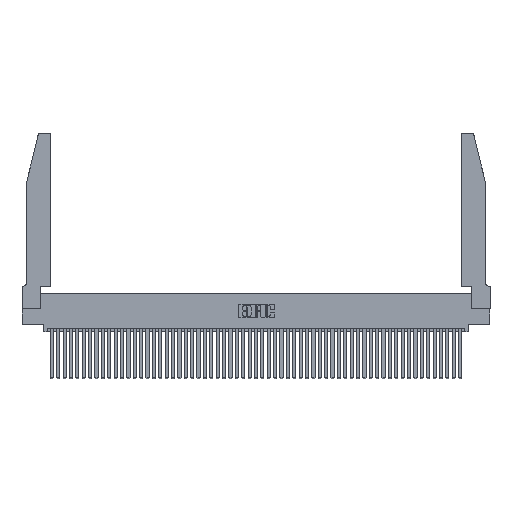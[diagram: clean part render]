
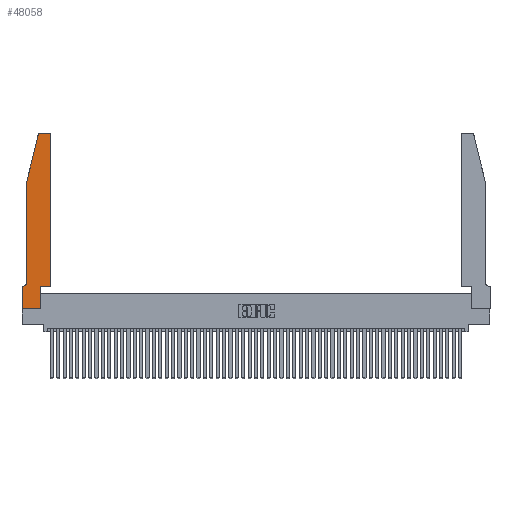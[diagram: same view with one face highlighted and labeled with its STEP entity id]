
A CAD part, top view. The second image highlights one B-rep face of the part: STEP entity #48058.
In plain terms, the highlighted planar face has unit normal (0, 0, 1).
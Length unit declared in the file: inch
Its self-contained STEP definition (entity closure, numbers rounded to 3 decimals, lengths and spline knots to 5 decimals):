
#108 = EDGE_CURVE ( 'NONE', #32407, #50588, #40248, .T. ) ;
#417 = DIRECTION ( 'NONE',  ( -1., 0., 0. ) ) ;
#1207 = EDGE_CURVE ( 'NONE', #45437, #23000, #37636, .T. ) ;
#2718 = DIRECTION ( 'NONE',  ( 1., 0., 0. ) ) ;
#3512 = CARTESIAN_POINT ( 'NONE',  ( 0.0755, 2., 0.37 ) ) ;
#3935 = VERTEX_POINT ( 'NONE', #17784 ) ;
#4068 = VECTOR ( 'NONE', #6669, 39.37008 ) ;
#4568 = DIRECTION ( 'NONE',  ( 0., 1., 0. ) ) ;
#4619 = ORIENTED_EDGE ( 'NONE', *, *, #37289, .T. ) ;
#4667 = VECTOR ( 'NONE', #39331, 39.37008 ) ;
#5758 = DIRECTION ( 'NONE',  ( 0., 0., 1. ) ) ;
#6669 = DIRECTION ( 'NONE',  ( -1., 0., 0. ) ) ;
#7235 = CARTESIAN_POINT ( 'NONE',  ( 0.0755, 0.35, 0.37 ) ) ;
#7594 = DIRECTION ( 'NONE',  ( -0.239, -0.971, 0. ) ) ;
#8000 = ORIENTED_EDGE ( 'NONE', *, *, #46721, .T. ) ;
#8265 = LINE ( 'NONE', #27307, #45809 ) ;
#9002 = LINE ( 'NONE', #36917, #34467 ) ;
#9204 = AXIS2_PLACEMENT_3D ( 'NONE', #42686, #26706, #26871 ) ;
#9353 = VECTOR ( 'NONE', #34110, 39.37008 ) ;
#9788 = LINE ( 'NONE', #3512, #52331 ) ;
#9932 = ORIENTED_EDGE ( 'NONE', *, *, #1207, .T. ) ;
#10025 = CARTESIAN_POINT ( 'NONE',  ( 0., 0., 0.37 ) ) ;
#11655 = CARTESIAN_POINT ( 'NONE',  ( 0.284, 2.75, 0.37 ) ) ;
#12198 = CARTESIAN_POINT ( 'NONE',  ( 0.0055, 0.42, 0.37 ) ) ;
#12377 = VERTEX_POINT ( 'NONE', #26930 ) ;
#12613 = EDGE_CURVE ( 'NONE', #50588, #3935, #20645, .T. ) ;
#12915 = CARTESIAN_POINT ( 'NONE',  ( 0.25487, 2.72718, 0.37 ) ) ;
#13933 = CARTESIAN_POINT ( 'NONE',  ( 0.2865, 0.35, 0.37 ) ) ;
#15765 = AXIS2_PLACEMENT_3D ( 'NONE', #12198, #24817, #417 ) ;
#15839 = ORIENTED_EDGE ( 'NONE', *, *, #20529, .T. ) ;
#17040 = EDGE_CURVE ( 'NONE', #39948, #32407, #26724, .T. ) ;
#17784 = CARTESIAN_POINT ( 'NONE',  ( 0.2865, 0., 0.37 ) ) ;
#18022 = AXIS2_PLACEMENT_3D ( 'NONE', #27081, #30800, #2718 ) ;
#18145 = CARTESIAN_POINT ( 'NONE',  ( 0.4205, 2.75, 0.37 ) ) ;
#19070 = PLANE ( 'NONE',  #18022 ) ;
#19079 = CARTESIAN_POINT ( 'NONE',  ( 0.2605, 2.75, 0.37 ) ) ;
#19269 = CARTESIAN_POINT ( 'NONE',  ( 0., 0., 0.37 ) ) ;
#20529 = EDGE_CURVE ( 'NONE', #36280, #29135, #9788, .T. ) ;
#20645 = LINE ( 'NONE', #19269, #34631 ) ;
#21589 = DIRECTION ( 'NONE',  ( 0., 1., 0. ) ) ;
#21901 = ORIENTED_EDGE ( 'NONE', *, *, #52190, .T. ) ;
#23000 = VERTEX_POINT ( 'NONE', #18145 ) ;
#23869 = CARTESIAN_POINT ( 'NONE',  ( 0.0755, 0.42, 0.37 ) ) ;
#24288 = CARTESIAN_POINT ( 'NONE',  ( 0.4505, 0.35, 0.37 ) ) ;
#24817 = DIRECTION ( 'NONE',  ( 0., 0., -1. ) ) ;
#26064 = VECTOR ( 'NONE', #51990, 39.37008 ) ;
#26697 = CARTESIAN_POINT ( 'NONE',  ( 0.284, 2.72, 0.37 ) ) ;
#26706 = DIRECTION ( 'NONE',  ( 0., 0., 1. ) ) ;
#26724 = LINE ( 'NONE', #7235, #26064 ) ;
#26871 = DIRECTION ( 'NONE',  ( 1., 0., 0. ) ) ;
#26930 = CARTESIAN_POINT ( 'NONE',  ( 0.2865, 0.35, 0.37 ) ) ;
#27081 = CARTESIAN_POINT ( 'NONE',  ( 0., 0.35, 0.37 ) ) ;
#27307 = CARTESIAN_POINT ( 'NONE',  ( 0.4505, 0.35, 0.37 ) ) ;
#27443 = DIRECTION ( 'NONE',  ( 1., 0., 0. ) ) ;
#28082 = ORIENTED_EDGE ( 'NONE', *, *, #108, .T. ) ;
#29135 = VERTEX_POINT ( 'NONE', #40677 ) ;
#29564 = CIRCLE ( 'NONE', #15765, 0.07 ) ;
#29857 = EDGE_CURVE ( 'NONE', #3935, #12377, #48520, .T. ) ;
#30345 = LINE ( 'NONE', #50435, #9353 ) ;
#30800 = DIRECTION ( 'NONE',  ( 0., 0., 1. ) ) ;
#31534 = DIRECTION ( 'NONE',  ( 1., 0., 0. ) ) ;
#32015 = CARTESIAN_POINT ( 'NONE',  ( 0.0055, 0.35, 0.37 ) ) ;
#32407 = VERTEX_POINT ( 'NONE', #50140 ) ;
#33489 = EDGE_CURVE ( 'NONE', #52221, #45437, #9002, .T. ) ;
#33830 = ORIENTED_EDGE ( 'NONE', *, *, #17040, .T. ) ;
#34055 = VERTEX_POINT ( 'NONE', #11655 ) ;
#34110 = DIRECTION ( 'NONE',  ( 0., -1., 0. ) ) ;
#34467 = VECTOR ( 'NONE', #4568, 39.37008 ) ;
#34631 = VECTOR ( 'NONE', #27443, 39.37008 ) ;
#35335 = CARTESIAN_POINT ( 'NONE',  ( 0.4505, 2.72, 0.37 ) ) ;
#36280 = VERTEX_POINT ( 'NONE', #12915 ) ;
#36613 = ORIENTED_EDGE ( 'NONE', *, *, #12613, .T. ) ;
#36917 = CARTESIAN_POINT ( 'NONE',  ( 0.4505, 0.35, 0.37 ) ) ;
#37289 = EDGE_CURVE ( 'NONE', #12377, #52221, #8265, .T. ) ;
#37447 = ORIENTED_EDGE ( 'NONE', *, *, #41580, .T. ) ;
#37636 = CIRCLE ( 'NONE', #9204, 0.03 ) ;
#38996 = EDGE_CURVE ( 'NONE', #29135, #39866, #30345, .T. ) ;
#39331 = DIRECTION ( 'NONE',  ( 0., -1., 0. ) ) ;
#39866 = VERTEX_POINT ( 'NONE', #23869 ) ;
#39929 = FACE_OUTER_BOUND ( 'NONE', #50922, .T. ) ;
#39948 = VERTEX_POINT ( 'NONE', #32015 ) ;
#40248 = LINE ( 'NONE', #10025, #4667 ) ;
#40677 = CARTESIAN_POINT ( 'NONE',  ( 0.0755, 2., 0.37 ) ) ;
#41580 = EDGE_CURVE ( 'NONE', #23000, #34055, #47903, .T. ) ;
#42201 = CARTESIAN_POINT ( 'NONE',  ( 0., 0., 0.37 ) ) ;
#42686 = CARTESIAN_POINT ( 'NONE',  ( 0.4205, 2.72, 0.37 ) ) ;
#43632 = ORIENTED_EDGE ( 'NONE', *, *, #33489, .T. ) ;
#44786 = ORIENTED_EDGE ( 'NONE', *, *, #38996, .T. ) ;
#45437 = VERTEX_POINT ( 'NONE', #35335 ) ;
#45809 = VECTOR ( 'NONE', #31534, 39.37008 ) ;
#46611 = DIRECTION ( 'NONE',  ( 1., 0., 0. ) ) ;
#46613 = AXIS2_PLACEMENT_3D ( 'NONE', #26697, #5758, #46611 ) ;
#46721 = EDGE_CURVE ( 'NONE', #34055, #36280, #49598, .T. ) ;
#47242 = ORIENTED_EDGE ( 'NONE', *, *, #29857, .T. ) ;
#47249 = VECTOR ( 'NONE', #21589, 39.37008 ) ;
#47903 = LINE ( 'NONE', #19079, #4068 ) ;
#48058 = ADVANCED_FACE ( 'NONE', ( #39929 ), #19070, .T. ) ;
#48520 = LINE ( 'NONE', #13933, #47249 ) ;
#49598 = CIRCLE ( 'NONE', #46613, 0.03 ) ;
#50140 = CARTESIAN_POINT ( 'NONE',  ( 0., 0.35, 0.37 ) ) ;
#50435 = CARTESIAN_POINT ( 'NONE',  ( 0.0755, 2., 0.37 ) ) ;
#50588 = VERTEX_POINT ( 'NONE', #42201 ) ;
#50922 = EDGE_LOOP ( 'NONE', ( #37447, #8000, #15839, #44786, #21901, #33830, #28082, #36613, #47242, #4619, #43632, #9932 ) ) ;
#51990 = DIRECTION ( 'NONE',  ( -1., 0., 0. ) ) ;
#52190 = EDGE_CURVE ( 'NONE', #39866, #39948, #29564, .T. ) ;
#52221 = VERTEX_POINT ( 'NONE', #24288 ) ;
#52331 = VECTOR ( 'NONE', #7594, 39.37008 ) ;
